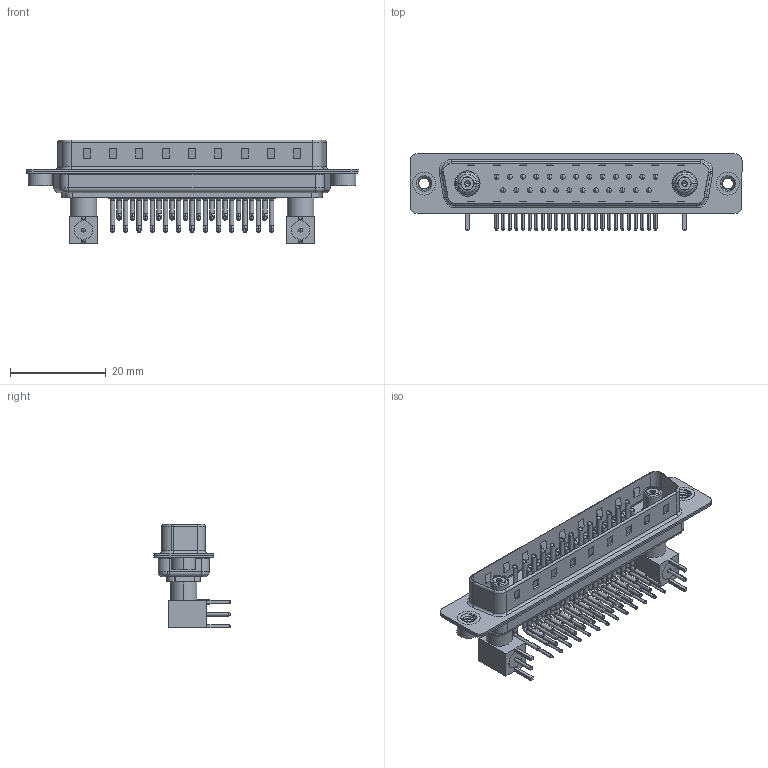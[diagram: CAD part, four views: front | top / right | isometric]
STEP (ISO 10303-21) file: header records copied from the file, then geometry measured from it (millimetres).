
FILE_DESCRIPTION (( 'STEP AP203' ), '1' );
FILE_NAME ('629-27W2640-7NA.STEP', '2022-05-16T20:06:07', ( '' ), ( '' ), 'SwSTEP 2.0', 'SolidWorks 2020', '' );
FILE_SCHEMA (( 'CONFIG_CONTROL_DESIGN' ));
Length unit declared in the file: millimetre
Products named in the file (16): Insulator Socket; 629Combo Shell Rear_37 Contacts; 629Combo Contact Row 2; Co-Ax Jack Assy_RA; Insulator Socket 2; Locking Collar; Insulator RA Pin; Socket_RA; 629Combo Contact Row 1; RA Back Shell; 629Combo Threaded Rivet_2; 629Combo Shell Front_37 Contacts; 629-27W2640-7NA; Co-Ax Jack_RA PC Tail; 629Combo Housing_27W2
Assembly tree (46 placements, depth 3):
  629-27W2640-7NA
    629Combo Housing_27W2
    629Combo Shell Rear_37 Contacts
    629Combo Shell Front_37 Contacts
    629Combo Threaded Rivet_2  x2
    Co-Ax Jack Assy_RA
      Co-Ax Jack_RA PC Tail
      Insulator Socket
      Insulator Socket 2
      Locking Collar
      Socket_RA
      RA Back Shell
      Insulator RA Pin
    Co-Ax Jack Assy_RA
      Co-Ax Jack_RA PC Tail
      Insulator Socket
      Insulator Socket 2
      Locking Collar
      Socket_RA
      RA Back Shell
      Insulator RA Pin
    629Combo Contact Row 1  x13
    629Combo Contact Row 2  x12
Bounding box: 69.4 x 16 x 21.71 mm (x, y, z)
Volume: 4535.7 mm3; surface area: 11790.4 mm2
Topology: 44 solids, 44 shells, 3466 faces, 9523 edges, 6168 vertices
Faces by surface type: plane 1917, cylinder 1175, bspline 158, cone 150, torus 62, sphere 4
Entity records: 32771 total; most frequent: CARTESIAN_POINT 6765, DIRECTION 5150, ORIENTED_EDGE 4698, EDGE_CURVE 2349, AXIS2_PLACEMENT_3D 1891, VERTEX_POINT 1515, LINE 1368, VECTOR 1368
